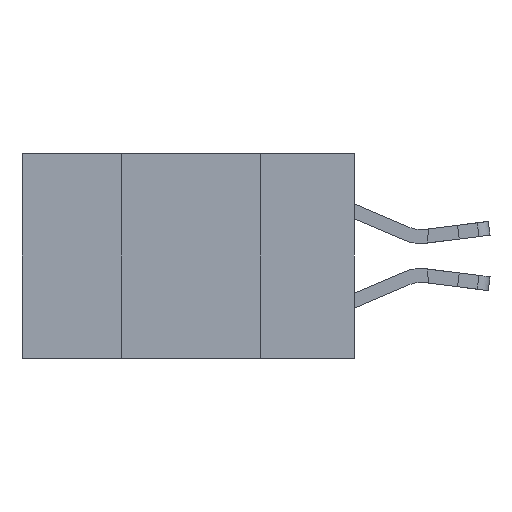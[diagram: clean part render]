
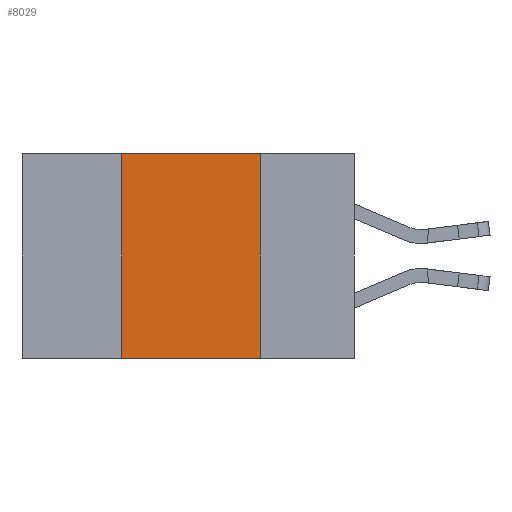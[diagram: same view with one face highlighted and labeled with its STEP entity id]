
A CAD part, left-side view. The second image highlights one B-rep face of the part: STEP entity #8029.
In plain terms, the highlighted planar face has unit normal (-1, 0, 0).
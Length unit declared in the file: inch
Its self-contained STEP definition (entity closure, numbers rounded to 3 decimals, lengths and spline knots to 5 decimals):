
#145 = ORIENTED_EDGE ( 'NONE', *, *, #6717, .F. ) ;
#337 = CARTESIAN_POINT ( 'NONE',  ( 0., 0.6, -0.37 ) ) ;
#838 = VECTOR ( 'NONE', #12197, 39.37008 ) ;
#1069 = EDGE_CURVE ( 'NONE', #9676, #4542, #12302, .T. ) ;
#1229 = CARTESIAN_POINT ( 'NONE',  ( 0., 0.6, 0. ) ) ;
#1505 = DIRECTION ( 'NONE',  ( 0., -1., 0. ) ) ;
#1554 = EDGE_CURVE ( 'NONE', #2813, #4542, #14462, .T. ) ;
#2434 = CARTESIAN_POINT ( 'NONE',  ( 0., 0.17, 0. ) ) ;
#2813 = VERTEX_POINT ( 'NONE', #2434 ) ;
#2939 = CARTESIAN_POINT ( 'NONE',  ( 0., 0.42, 0. ) ) ;
#3105 = CARTESIAN_POINT ( 'NONE',  ( 0., 0.6, 0. ) ) ;
#3863 = VERTEX_POINT ( 'NONE', #4363 ) ;
#4363 = CARTESIAN_POINT ( 'NONE',  ( 0., 0.42, 0. ) ) ;
#4542 = VERTEX_POINT ( 'NONE', #7274 ) ;
#4803 = DIRECTION ( 'NONE',  ( 0., -1., 0. ) ) ;
#5237 = ORIENTED_EDGE ( 'NONE', *, *, #14439, .F. ) ;
#5275 = VECTOR ( 'NONE', #4803, 39.37008 ) ;
#5427 = EDGE_LOOP ( 'NONE', ( #8957, #5237, #145, #6972 ) ) ;
#5866 = DIRECTION ( 'NONE',  ( 0., 0., -1. ) ) ;
#6624 = CARTESIAN_POINT ( 'NONE',  ( 0., 0.42, -0.37 ) ) ;
#6717 = EDGE_CURVE ( 'NONE', #9676, #3863, #11867, .T. ) ;
#6972 = ORIENTED_EDGE ( 'NONE', *, *, #1069, .T. ) ;
#7274 = CARTESIAN_POINT ( 'NONE',  ( 0., 0.17, -0.37 ) ) ;
#8029 = ADVANCED_FACE ( 'NONE', ( #13458 ), #8680, .F. ) ;
#8680 = PLANE ( 'NONE',  #12778 ) ;
#8837 = DIRECTION ( 'NONE',  ( 1., 0., 0. ) ) ;
#8957 = ORIENTED_EDGE ( 'NONE', *, *, #1554, .F. ) ;
#9676 = VERTEX_POINT ( 'NONE', #6624 ) ;
#10027 = DIRECTION ( 'NONE',  ( 0., 0., -1. ) ) ;
#11867 = LINE ( 'NONE', #2939, #838 ) ;
#12197 = DIRECTION ( 'NONE',  ( 0., 0., 1. ) ) ;
#12293 = VECTOR ( 'NONE', #5866, 39.37008 ) ;
#12302 = LINE ( 'NONE', #337, #14113 ) ;
#12775 = CARTESIAN_POINT ( 'NONE',  ( 0., 0.17, 0. ) ) ;
#12778 = AXIS2_PLACEMENT_3D ( 'NONE', #3105, #8837, #10027 ) ;
#13413 = LINE ( 'NONE', #1229, #5275 ) ;
#13458 = FACE_OUTER_BOUND ( 'NONE', #5427, .T. ) ;
#14113 = VECTOR ( 'NONE', #1505, 39.37008 ) ;
#14439 = EDGE_CURVE ( 'NONE', #3863, #2813, #13413, .T. ) ;
#14462 = LINE ( 'NONE', #12775, #12293 ) ;
